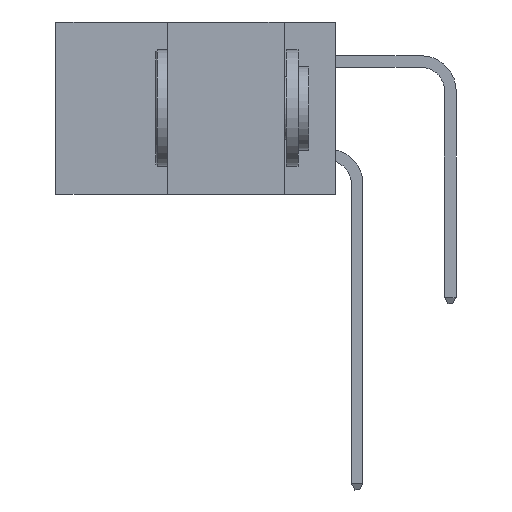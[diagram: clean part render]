
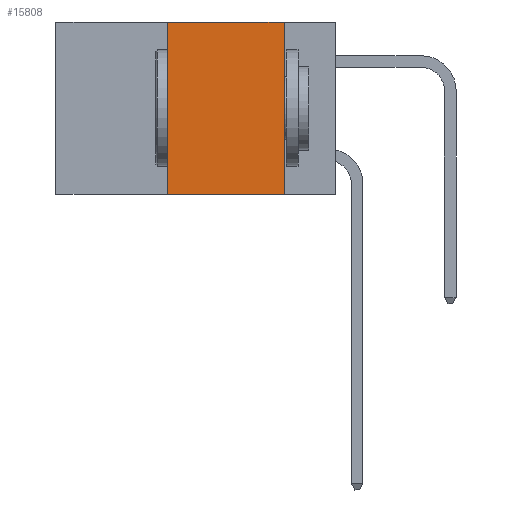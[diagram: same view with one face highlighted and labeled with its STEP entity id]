
A CAD part, left-side view. The second image highlights one B-rep face of the part: STEP entity #15808.
In plain terms, the highlighted planar face has unit normal (-1, 0, 0).
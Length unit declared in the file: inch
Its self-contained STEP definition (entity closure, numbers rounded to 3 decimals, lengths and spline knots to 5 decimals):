
#1305 = VERTEX_POINT ( 'NONE', #25937 ) ;
#2150 = ORIENTED_EDGE ( 'NONE', *, *, #14539, .T. ) ;
#2531 = CARTESIAN_POINT ( 'NONE',  ( 0., 0.36, 0. ) ) ;
#2619 = ORIENTED_EDGE ( 'NONE', *, *, #25948, .F. ) ;
#3591 = VERTEX_POINT ( 'NONE', #13808 ) ;
#3715 = CARTESIAN_POINT ( 'NONE',  ( 0., 0.36, 0. ) ) ;
#3963 = DIRECTION ( 'NONE',  ( 0., 0., -1. ) ) ;
#6730 = ORIENTED_EDGE ( 'NONE', *, *, #22472, .F. ) ;
#7286 = EDGE_LOOP ( 'NONE', ( #2619, #6730, #19976, #2150 ) ) ;
#7904 = FACE_OUTER_BOUND ( 'NONE', #7286, .T. ) ;
#9127 = PLANE ( 'NONE',  #9838 ) ;
#9554 = CARTESIAN_POINT ( 'NONE',  ( 0., 0.6, 0. ) ) ;
#9793 = CARTESIAN_POINT ( 'NONE',  ( 0., 0.11, 0. ) ) ;
#9838 = AXIS2_PLACEMENT_3D ( 'NONE', #24328, #15555, #11537 ) ;
#9914 = VECTOR ( 'NONE', #24518, 39.37008 ) ;
#11411 = VECTOR ( 'NONE', #18697, 39.37008 ) ;
#11537 = DIRECTION ( 'NONE',  ( 0., 0., -1. ) ) ;
#13808 = CARTESIAN_POINT ( 'NONE',  ( 0., 0.11, -0.37 ) ) ;
#14220 = DIRECTION ( 'NONE',  ( 0., -1., 0. ) ) ;
#14539 = EDGE_CURVE ( 'NONE', #1305, #3591, #16343, .T. ) ;
#14990 = LINE ( 'NONE', #25388, #18008 ) ;
#15245 = VERTEX_POINT ( 'NONE', #2531 ) ;
#15266 = LINE ( 'NONE', #9554, #9914 ) ;
#15555 = DIRECTION ( 'NONE',  ( 1., 0., 0. ) ) ;
#15808 = ADVANCED_FACE ( 'NONE', ( #7904 ), #9127, .F. ) ;
#16343 = LINE ( 'NONE', #16450, #19360 ) ;
#16450 = CARTESIAN_POINT ( 'NONE',  ( 0., 0.6, -0.37 ) ) ;
#18008 = VECTOR ( 'NONE', #3963, 39.37008 ) ;
#18697 = DIRECTION ( 'NONE',  ( 0., 0., 1. ) ) ;
#19360 = VECTOR ( 'NONE', #14220, 39.37008 ) ;
#19976 = ORIENTED_EDGE ( 'NONE', *, *, #24429, .F. ) ;
#22472 = EDGE_CURVE ( 'NONE', #15245, #24280, #15266, .T. ) ;
#23772 = LINE ( 'NONE', #3715, #11411 ) ;
#24280 = VERTEX_POINT ( 'NONE', #9793 ) ;
#24328 = CARTESIAN_POINT ( 'NONE',  ( 0., 0.6, 0. ) ) ;
#24429 = EDGE_CURVE ( 'NONE', #1305, #15245, #23772, .T. ) ;
#24518 = DIRECTION ( 'NONE',  ( 0., -1., 0. ) ) ;
#25388 = CARTESIAN_POINT ( 'NONE',  ( 0., 0.11, 0. ) ) ;
#25937 = CARTESIAN_POINT ( 'NONE',  ( 0., 0.36, -0.37 ) ) ;
#25948 = EDGE_CURVE ( 'NONE', #24280, #3591, #14990, .T. ) ;
